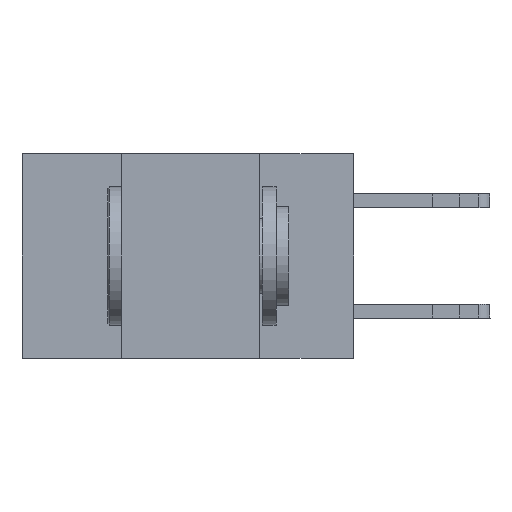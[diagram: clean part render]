
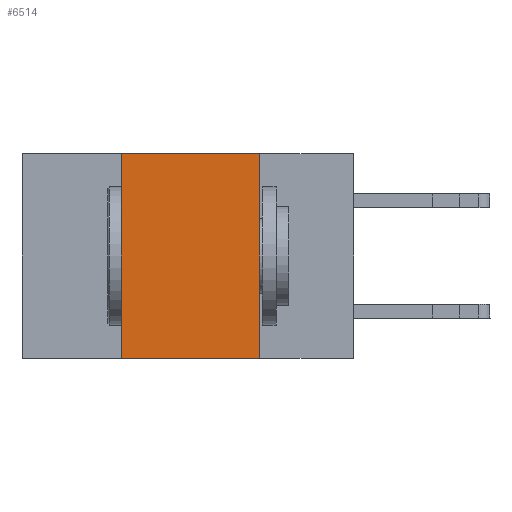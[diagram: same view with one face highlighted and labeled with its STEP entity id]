
A CAD part, left-side view. The second image highlights one B-rep face of the part: STEP entity #6514.
In plain terms, the highlighted planar face has unit normal (-1, 0, 0).
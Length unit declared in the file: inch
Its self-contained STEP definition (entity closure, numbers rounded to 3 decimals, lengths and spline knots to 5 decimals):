
#97 = CARTESIAN_POINT ( 'NONE',  ( 0., 0.42, -0.37 ) ) ;
#525 = VECTOR ( 'NONE', #6185, 39.37008 ) ;
#649 = VECTOR ( 'NONE', #4944, 39.37008 ) ;
#1245 = PLANE ( 'NONE',  #1258 ) ;
#1258 = AXIS2_PLACEMENT_3D ( 'NONE', #10631, #17348, #9399 ) ;
#1885 = VECTOR ( 'NONE', #15434, 39.37008 ) ;
#2472 = VERTEX_POINT ( 'NONE', #8923 ) ;
#2708 = EDGE_CURVE ( 'NONE', #2472, #10757, #4245, .T. ) ;
#2753 = ORIENTED_EDGE ( 'NONE', *, *, #4885, .F. ) ;
#3909 = EDGE_LOOP ( 'NONE', ( #16552, #2753, #16185, #14298 ) ) ;
#4245 = LINE ( 'NONE', #6173, #525 ) ;
#4811 = LINE ( 'NONE', #12815, #649 ) ;
#4885 = EDGE_CURVE ( 'NONE', #5565, #2472, #15579, .T. ) ;
#4944 = DIRECTION ( 'NONE',  ( 0., -1., 0. ) ) ;
#5565 = VERTEX_POINT ( 'NONE', #11462 ) ;
#6173 = CARTESIAN_POINT ( 'NONE',  ( 0., 0.17, 0. ) ) ;
#6185 = DIRECTION ( 'NONE',  ( 0., 0., -1. ) ) ;
#6514 = ADVANCED_FACE ( 'NONE', ( #6656 ), #1245, .F. ) ;
#6656 = FACE_OUTER_BOUND ( 'NONE', #3909, .T. ) ;
#7139 = VERTEX_POINT ( 'NONE', #97 ) ;
#8123 = EDGE_CURVE ( 'NONE', #7139, #5565, #12122, .T. ) ;
#8923 = CARTESIAN_POINT ( 'NONE',  ( 0., 0.17, 0. ) ) ;
#9399 = DIRECTION ( 'NONE',  ( 0., 0., -1. ) ) ;
#9874 = EDGE_CURVE ( 'NONE', #7139, #10757, #4811, .T. ) ;
#10631 = CARTESIAN_POINT ( 'NONE',  ( 0., 0.6, 0. ) ) ;
#10757 = VERTEX_POINT ( 'NONE', #15036 ) ;
#11462 = CARTESIAN_POINT ( 'NONE',  ( 0., 0.42, 0. ) ) ;
#12038 = VECTOR ( 'NONE', #15714, 39.37008 ) ;
#12122 = LINE ( 'NONE', #14082, #1885 ) ;
#12815 = CARTESIAN_POINT ( 'NONE',  ( 0., 0.6, -0.37 ) ) ;
#14082 = CARTESIAN_POINT ( 'NONE',  ( 0., 0.42, 0. ) ) ;
#14298 = ORIENTED_EDGE ( 'NONE', *, *, #9874, .T. ) ;
#15036 = CARTESIAN_POINT ( 'NONE',  ( 0., 0.17, -0.37 ) ) ;
#15434 = DIRECTION ( 'NONE',  ( 0., 0., 1. ) ) ;
#15579 = LINE ( 'NONE', #16321, #12038 ) ;
#15714 = DIRECTION ( 'NONE',  ( 0., -1., 0. ) ) ;
#16185 = ORIENTED_EDGE ( 'NONE', *, *, #8123, .F. ) ;
#16321 = CARTESIAN_POINT ( 'NONE',  ( 0., 0.6, 0. ) ) ;
#16552 = ORIENTED_EDGE ( 'NONE', *, *, #2708, .F. ) ;
#17348 = DIRECTION ( 'NONE',  ( 1., 0., 0. ) ) ;
